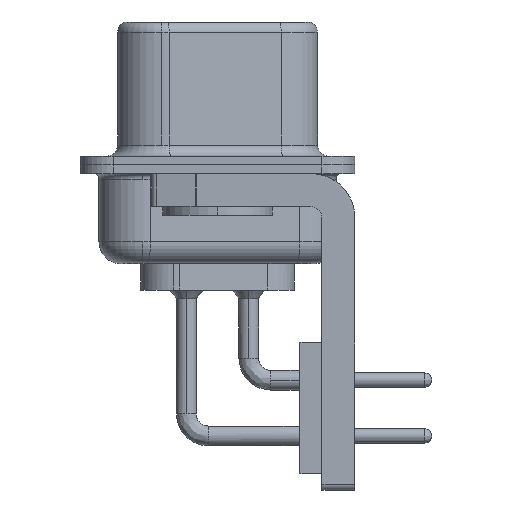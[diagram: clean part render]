
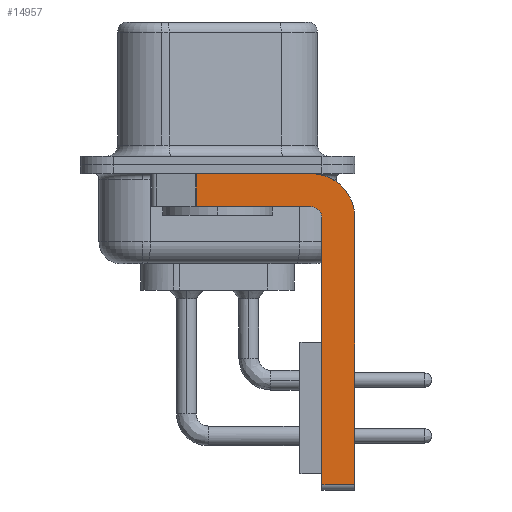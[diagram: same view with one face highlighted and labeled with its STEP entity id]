
A CAD part, left-side view. The second image highlights one B-rep face of the part: STEP entity #14957.
In plain terms, the highlighted planar face has unit normal (-1, 0, 0).
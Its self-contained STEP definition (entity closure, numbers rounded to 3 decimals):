
#457 = DIRECTION ( 'NONE',  ( 0., -1., 0. ) ) ;
#936 = VERTEX_POINT ( 'NONE', #12968 ) ;
#1398 = ORIENTED_EDGE ( 'NONE', *, *, #5523, .T. ) ;
#1592 = VECTOR ( 'NONE', #22609, 1000. ) ;
#1764 = EDGE_CURVE ( 'NONE', #12503, #23047, #2217, .T. ) ;
#2076 = DIRECTION ( 'NONE',  ( 0., 0., -1. ) ) ;
#2160 = CARTESIAN_POINT ( 'NONE',  ( -2.9, 0.978, -1.9 ) ) ;
#2217 = LINE ( 'NONE', #17491, #17356 ) ;
#3150 = CARTESIAN_POINT ( 'NONE',  ( -2.9, -4.25, -0.4 ) ) ;
#3364 = AXIS2_PLACEMENT_3D ( 'NONE', #10405, #23366, #12317 ) ;
#4609 = ORIENTED_EDGE ( 'NONE', *, *, #21750, .F. ) ;
#4653 = PLANE ( 'NONE',  #4708 ) ;
#4708 = AXIS2_PLACEMENT_3D ( 'NONE', #17825, #19686, #8483 ) ;
#4950 = VERTEX_POINT ( 'NONE', #12831 ) ;
#5218 = VERTEX_POINT ( 'NONE', #6925 ) ;
#5523 = EDGE_CURVE ( 'NONE', #8670, #4950, #6342, .T. ) ;
#5753 = VECTOR ( 'NONE', #2076, 1000. ) ;
#6342 = LINE ( 'NONE', #2160, #5753 ) ;
#6477 = EDGE_CURVE ( 'NONE', #15611, #23047, #16900, .T. ) ;
#6848 = CARTESIAN_POINT ( 'NONE',  ( -2.9, -4.25, -2.4 ) ) ;
#6925 = CARTESIAN_POINT ( 'NONE',  ( -2.9, -4.75, -2.4 ) ) ;
#7262 = DIRECTION ( 'NONE',  ( 0., 1., 0. ) ) ;
#7465 = VECTOR ( 'NONE', #20320, 1000. ) ;
#7657 = ORIENTED_EDGE ( 'NONE', *, *, #22759, .F. ) ;
#7920 = LINE ( 'NONE', #20528, #8535 ) ;
#8309 = CARTESIAN_POINT ( 'NONE',  ( -2.9, -6.25, -14.55 ) ) ;
#8483 = DIRECTION ( 'NONE',  ( 0., 0., -1. ) ) ;
#8535 = VECTOR ( 'NONE', #7262, 1000. ) ;
#8670 = VERTEX_POINT ( 'NONE', #12536 ) ;
#8781 = DIRECTION ( 'NONE',  ( 0., 0., -1. ) ) ;
#9585 = CARTESIAN_POINT ( 'NONE',  ( -2.9, -4.75, -14.8 ) ) ;
#9649 = DIRECTION ( 'NONE',  ( 0., -1., 0. ) ) ;
#10405 = CARTESIAN_POINT ( 'NONE',  ( -2.9, -4.25, -2.4 ) ) ;
#11505 = EDGE_LOOP ( 'NONE', ( #13759, #1398, #18048, #4609, #7657, #13621, #20567, #21383 ) ) ;
#11593 = AXIS2_PLACEMENT_3D ( 'NONE', #6848, #19966, #8781 ) ;
#12317 = DIRECTION ( 'NONE',  ( 0., 0., 1. ) ) ;
#12404 = LINE ( 'NONE', #9585, #1592 ) ;
#12503 = VERTEX_POINT ( 'NONE', #16077 ) ;
#12536 = CARTESIAN_POINT ( 'NONE',  ( -2.9, 0.978, -0.4 ) ) ;
#12685 = LINE ( 'NONE', #22669, #21947 ) ;
#12831 = CARTESIAN_POINT ( 'NONE',  ( -2.9, 0.978, -1.9 ) ) ;
#12968 = CARTESIAN_POINT ( 'NONE',  ( -2.9, -4.25, -1.9 ) ) ;
#13621 = ORIENTED_EDGE ( 'NONE', *, *, #1764, .T. ) ;
#13759 = ORIENTED_EDGE ( 'NONE', *, *, #21494, .F. ) ;
#14957 = ADVANCED_FACE ( 'NONE', ( #16160 ), #4653, .F. ) ;
#15611 = VERTEX_POINT ( 'NONE', #21736 ) ;
#16077 = CARTESIAN_POINT ( 'NONE',  ( -2.9, -4.75, -14.55 ) ) ;
#16160 = FACE_OUTER_BOUND ( 'NONE', #11505, .T. ) ;
#16725 = CIRCLE ( 'NONE', #11593, 2. ) ;
#16900 = LINE ( 'NONE', #20274, #7465 ) ;
#17064 = CIRCLE ( 'NONE', #3364, 0.5 ) ;
#17356 = VECTOR ( 'NONE', #457, 1000. ) ;
#17491 = CARTESIAN_POINT ( 'NONE',  ( -2.9, -4.25, -14.55 ) ) ;
#17825 = CARTESIAN_POINT ( 'NONE',  ( -2.9, -4.25, -2.4 ) ) ;
#18048 = ORIENTED_EDGE ( 'NONE', *, *, #22705, .F. ) ;
#19686 = DIRECTION ( 'NONE',  ( 1., 0., 0. ) ) ;
#19966 = DIRECTION ( 'NONE',  ( 1., 0., 0. ) ) ;
#20256 = VERTEX_POINT ( 'NONE', #3150 ) ;
#20274 = CARTESIAN_POINT ( 'NONE',  ( -2.9, -6.25, -2.4 ) ) ;
#20320 = DIRECTION ( 'NONE',  ( 0., 0., -1. ) ) ;
#20528 = CARTESIAN_POINT ( 'NONE',  ( -2.9, -4.25, -1.9 ) ) ;
#20567 = ORIENTED_EDGE ( 'NONE', *, *, #6477, .F. ) ;
#21383 = ORIENTED_EDGE ( 'NONE', *, *, #23699, .F. ) ;
#21494 = EDGE_CURVE ( 'NONE', #8670, #20256, #12685, .T. ) ;
#21736 = CARTESIAN_POINT ( 'NONE',  ( -2.9, -6.25, -2.4 ) ) ;
#21750 = EDGE_CURVE ( 'NONE', #5218, #936, #17064, .T. ) ;
#21947 = VECTOR ( 'NONE', #9649, 1000. ) ;
#22609 = DIRECTION ( 'NONE',  ( 0., 0., 1. ) ) ;
#22669 = CARTESIAN_POINT ( 'NONE',  ( -2.9, 3., -0.4 ) ) ;
#22705 = EDGE_CURVE ( 'NONE', #936, #4950, #7920, .T. ) ;
#22759 = EDGE_CURVE ( 'NONE', #12503, #5218, #12404, .T. ) ;
#23047 = VERTEX_POINT ( 'NONE', #8309 ) ;
#23366 = DIRECTION ( 'NONE',  ( -1., 0., 0. ) ) ;
#23699 = EDGE_CURVE ( 'NONE', #20256, #15611, #16725, .T. ) ;
